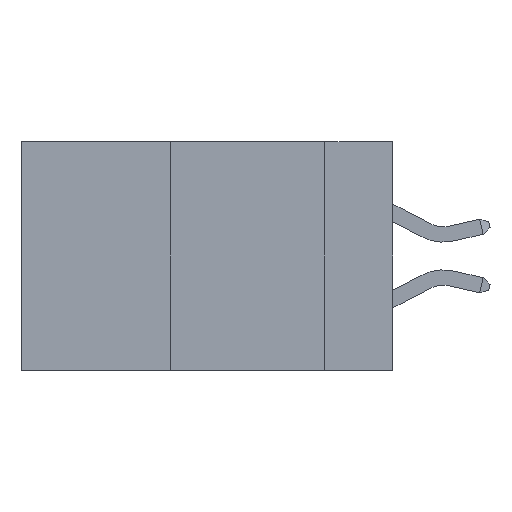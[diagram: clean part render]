
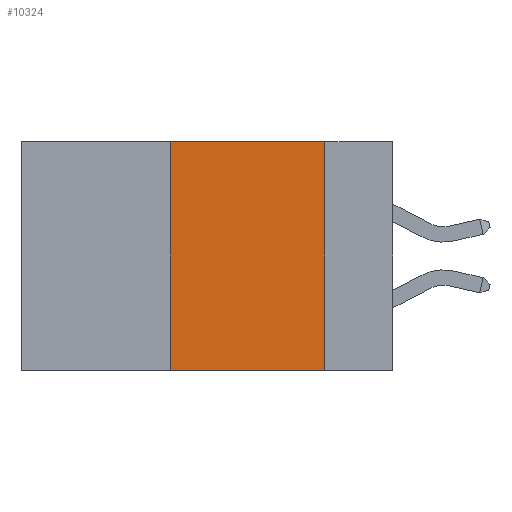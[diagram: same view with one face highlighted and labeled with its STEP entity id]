
A CAD part, left-side view. The second image highlights one B-rep face of the part: STEP entity #10324.
In plain terms, the highlighted planar face has unit normal (-1, 0, 0).
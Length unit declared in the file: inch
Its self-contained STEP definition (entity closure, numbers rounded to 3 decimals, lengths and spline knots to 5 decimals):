
#105 = LINE ( 'NONE', #5634, #11140 ) ;
#547 = VECTOR ( 'NONE', #13749, 39.37008 ) ;
#1006 = DIRECTION ( 'NONE',  ( 0., -1., 0. ) ) ;
#1588 = VERTEX_POINT ( 'NONE', #3305 ) ;
#1628 = CARTESIAN_POINT ( 'NONE',  ( 0., 0.11, -0.37 ) ) ;
#2341 = CARTESIAN_POINT ( 'NONE',  ( 0., 0.6, 0. ) ) ;
#3305 = CARTESIAN_POINT ( 'NONE',  ( 0., 0.36, 0. ) ) ;
#3624 = VERTEX_POINT ( 'NONE', #1628 ) ;
#4205 = VECTOR ( 'NONE', #15391, 39.37008 ) ;
#5005 = CARTESIAN_POINT ( 'NONE',  ( 0., 0.36, -0.37 ) ) ;
#5634 = CARTESIAN_POINT ( 'NONE',  ( 0., 0.11, 0. ) ) ;
#5857 = VERTEX_POINT ( 'NONE', #5005 ) ;
#6525 = PLANE ( 'NONE',  #11627 ) ;
#6580 = EDGE_CURVE ( 'NONE', #5857, #3624, #8662, .T. ) ;
#7586 = ORIENTED_EDGE ( 'NONE', *, *, #15101, .F. ) ;
#8600 = DIRECTION ( 'NONE',  ( 0., 0., -1. ) ) ;
#8662 = LINE ( 'NONE', #13447, #25078 ) ;
#9178 = ORIENTED_EDGE ( 'NONE', *, *, #16907, .F. ) ;
#9674 = LINE ( 'NONE', #19443, #4205 ) ;
#10004 = ORIENTED_EDGE ( 'NONE', *, *, #6580, .T. ) ;
#10324 = ADVANCED_FACE ( 'NONE', ( #16239 ), #6525, .F. ) ;
#11140 = VECTOR ( 'NONE', #17974, 39.37008 ) ;
#11627 = AXIS2_PLACEMENT_3D ( 'NONE', #2341, #20948, #8600 ) ;
#11660 = CARTESIAN_POINT ( 'NONE',  ( 0., 0.6, 0. ) ) ;
#12849 = VERTEX_POINT ( 'NONE', #25037 ) ;
#13447 = CARTESIAN_POINT ( 'NONE',  ( 0., 0.6, -0.37 ) ) ;
#13749 = DIRECTION ( 'NONE',  ( 0., -1., 0. ) ) ;
#15101 = EDGE_CURVE ( 'NONE', #12849, #3624, #105, .T. ) ;
#15391 = DIRECTION ( 'NONE',  ( 0., 0., 1. ) ) ;
#16239 = FACE_OUTER_BOUND ( 'NONE', #24723, .T. ) ;
#16907 = EDGE_CURVE ( 'NONE', #1588, #12849, #17077, .T. ) ;
#17077 = LINE ( 'NONE', #11660, #547 ) ;
#17974 = DIRECTION ( 'NONE',  ( 0., 0., -1. ) ) ;
#19443 = CARTESIAN_POINT ( 'NONE',  ( 0., 0.36, 0. ) ) ;
#19672 = ORIENTED_EDGE ( 'NONE', *, *, #24517, .F. ) ;
#20948 = DIRECTION ( 'NONE',  ( 1., 0., 0. ) ) ;
#24517 = EDGE_CURVE ( 'NONE', #5857, #1588, #9674, .T. ) ;
#24723 = EDGE_LOOP ( 'NONE', ( #7586, #9178, #19672, #10004 ) ) ;
#25037 = CARTESIAN_POINT ( 'NONE',  ( 0., 0.11, 0. ) ) ;
#25078 = VECTOR ( 'NONE', #1006, 39.37008 ) ;
